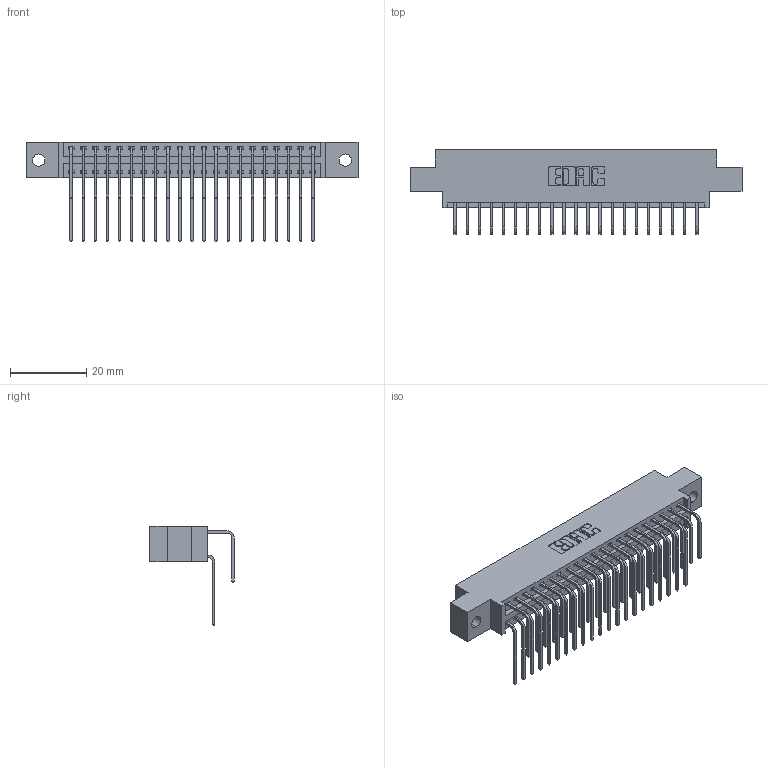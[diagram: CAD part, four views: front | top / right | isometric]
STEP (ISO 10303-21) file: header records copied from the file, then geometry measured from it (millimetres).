
FILE_DESCRIPTION (( 'STEP AP203' ), '1' );
FILE_NAME ('396-042-558-802.STEP', '2018-09-07T01:19:31', ( '' ), ( '' ), 'SwSTEP 2.0', 'SolidWorks 2016', '' );
FILE_SCHEMA (( 'CONFIG_CONTROL_DESIGN' ));
Length unit declared in the file: inch
Products named in the file (4): 346 Part_0.170 Offset - 0.128 Dia; 345-292-001_558 559 Tail - 1; 345-292-001_558 Tail - 2; 396-042-558-802
Assembly tree (43 placements, depth 2):
  396-042-558-802
    346 Part_0.170 Offset - 0.128 Dia
    345-292-001_558 559 Tail - 1  x21
    345-292-001_558 Tail - 2  x21
Bounding box: 87.25 x 22.16 x 26.16 mm (x, y, z)
Volume: 8395.7 mm3; surface area: 12283.2 mm2
Topology: 43 solids, 43 shells, 2394 faces, 7103 edges, 4678 vertices
Faces by surface type: plane 1634, cylinder 760
Entity records: 18451 total; most frequent: CARTESIAN_POINT 3123, ORIENTED_EDGE 3006, DIRECTION 2775, EDGE_CURVE 1503, VECTOR 1247, LINE 1247, VERTEX_POINT 998, AXIS2_PLACEMENT_3D 764
